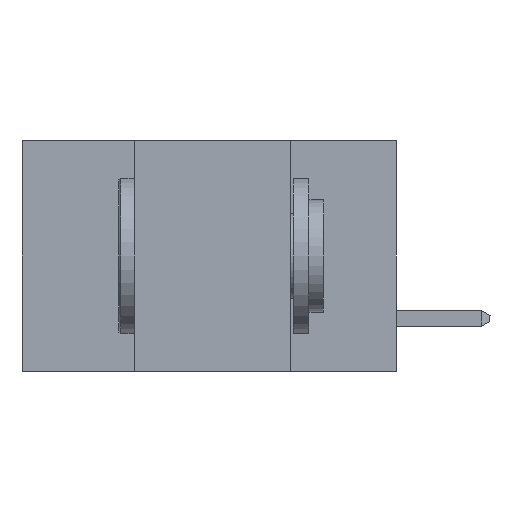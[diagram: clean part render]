
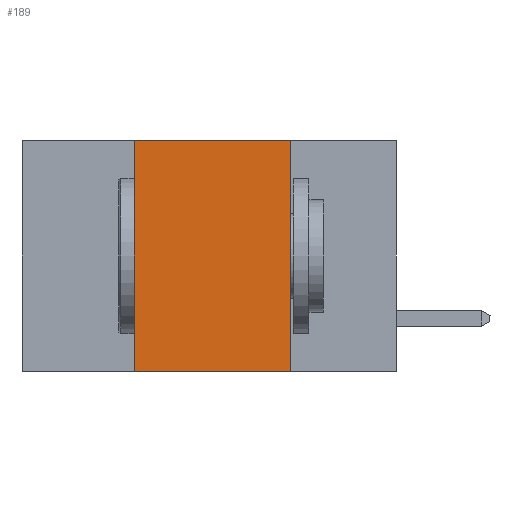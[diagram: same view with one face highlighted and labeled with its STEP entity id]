
A CAD part, left-side view. The second image highlights one B-rep face of the part: STEP entity #189.
In plain terms, the highlighted planar face has unit normal (-1, 0, 0).
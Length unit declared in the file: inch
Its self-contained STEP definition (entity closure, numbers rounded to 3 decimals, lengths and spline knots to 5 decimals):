
#189 = ADVANCED_FACE ( 'NONE', ( #10575 ), #19942, .F. ) ;
#1346 = EDGE_CURVE ( 'NONE', #15104, #5118, #8593, .T. ) ;
#3320 = CARTESIAN_POINT ( 'NONE',  ( 0., 0.17, -0.37 ) ) ;
#3434 = DIRECTION ( 'NONE',  ( 1., 0., 0. ) ) ;
#3881 = CARTESIAN_POINT ( 'NONE',  ( 0., 0.17, -0.37 ) ) ;
#3907 = CARTESIAN_POINT ( 'NONE',  ( 0., 0.6, 0. ) ) ;
#4702 = EDGE_CURVE ( 'NONE', #17379, #11978, #17641, .T. ) ;
#5118 = VERTEX_POINT ( 'NONE', #3881 ) ;
#5378 = VECTOR ( 'NONE', #12112, 39.37008 ) ;
#6276 = EDGE_CURVE ( 'NONE', #17379, #5118, #20489, .T. ) ;
#7210 = DIRECTION ( 'NONE',  ( 0., 0., 1. ) ) ;
#7729 = ORIENTED_EDGE ( 'NONE', *, *, #1346, .F. ) ;
#7742 = CARTESIAN_POINT ( 'NONE',  ( 0., 0.17, 0. ) ) ;
#8366 = VECTOR ( 'NONE', #17550, 39.37008 ) ;
#8593 = LINE ( 'NONE', #3320, #5378 ) ;
#8899 = CARTESIAN_POINT ( 'NONE',  ( 0., 0.42, 0. ) ) ;
#9090 = EDGE_CURVE ( 'NONE', #11978, #15104, #11926, .T. ) ;
#9788 = CARTESIAN_POINT ( 'NONE',  ( 0., 0.42, -0.37 ) ) ;
#9943 = DIRECTION ( 'NONE',  ( 0., -1., 0. ) ) ;
#10575 = FACE_OUTER_BOUND ( 'NONE', #20664, .T. ) ;
#10720 = CARTESIAN_POINT ( 'NONE',  ( 0., 0.42, -0.37 ) ) ;
#11926 = LINE ( 'NONE', #19069, #8366 ) ;
#11978 = VERTEX_POINT ( 'NONE', #8899 ) ;
#12112 = DIRECTION ( 'NONE',  ( 0., 0., -1. ) ) ;
#12452 = AXIS2_PLACEMENT_3D ( 'NONE', #3907, #3434, #21576 ) ;
#13009 = VECTOR ( 'NONE', #9943, 39.37008 ) ;
#14879 = CARTESIAN_POINT ( 'NONE',  ( 0., 0.6, -0.37 ) ) ;
#15104 = VERTEX_POINT ( 'NONE', #7742 ) ;
#15312 = VECTOR ( 'NONE', #7210, 39.37008 ) ;
#16041 = ORIENTED_EDGE ( 'NONE', *, *, #6276, .T. ) ;
#17379 = VERTEX_POINT ( 'NONE', #9788 ) ;
#17550 = DIRECTION ( 'NONE',  ( 0., -1., 0. ) ) ;
#17641 = LINE ( 'NONE', #10720, #15312 ) ;
#19069 = CARTESIAN_POINT ( 'NONE',  ( 0., 0.6, 0. ) ) ;
#19942 = PLANE ( 'NONE',  #12452 ) ;
#20489 = LINE ( 'NONE', #14879, #13009 ) ;
#20652 = ORIENTED_EDGE ( 'NONE', *, *, #4702, .F. ) ;
#20664 = EDGE_LOOP ( 'NONE', ( #7729, #20987, #20652, #16041 ) ) ;
#20987 = ORIENTED_EDGE ( 'NONE', *, *, #9090, .F. ) ;
#21576 = DIRECTION ( 'NONE',  ( 0., 0., -1. ) ) ;
